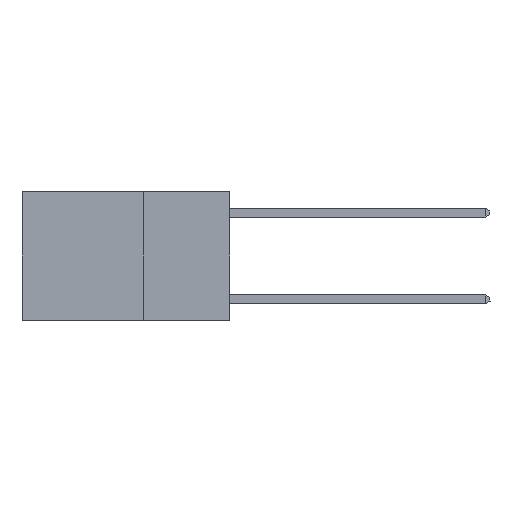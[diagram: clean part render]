
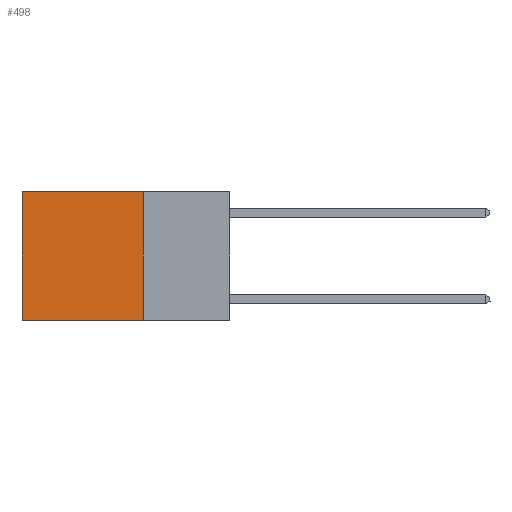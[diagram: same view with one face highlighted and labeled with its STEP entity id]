
A CAD part, left-side view. The second image highlights one B-rep face of the part: STEP entity #498.
In plain terms, the highlighted planar face has unit normal (-1, 0, 0).
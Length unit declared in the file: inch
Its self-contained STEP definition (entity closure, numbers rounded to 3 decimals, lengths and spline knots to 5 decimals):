
#197 = DIRECTION ( 'NONE',  ( 0., 1., 0. ) ) ;
#498 = ADVANCED_FACE ( 'NONE', ( #17595 ), #15581, .F. ) ;
#2174 = EDGE_CURVE ( 'NONE', #12027, #7402, #4754, .T. ) ;
#3318 = LINE ( 'NONE', #11327, #19541 ) ;
#3967 = ORIENTED_EDGE ( 'NONE', *, *, #12951, .T. ) ;
#4261 = VECTOR ( 'NONE', #20274, 39.37008 ) ;
#4628 = VERTEX_POINT ( 'NONE', #7171 ) ;
#4754 = LINE ( 'NONE', #18707, #4261 ) ;
#5888 = AXIS2_PLACEMENT_3D ( 'NONE', #7722, #9284, #20258 ) ;
#7171 = CARTESIAN_POINT ( 'NONE',  ( 0.2625, 0.6, -0.37 ) ) ;
#7172 = VERTEX_POINT ( 'NONE', #12004 ) ;
#7402 = VERTEX_POINT ( 'NONE', #12415 ) ;
#7722 = CARTESIAN_POINT ( 'NONE',  ( 0.2625, 0.25, 0. ) ) ;
#7856 = LINE ( 'NONE', #9628, #12034 ) ;
#8033 = EDGE_CURVE ( 'NONE', #7402, #4628, #13381, .T. ) ;
#9284 = DIRECTION ( 'NONE',  ( 1., 0., 0. ) ) ;
#9628 = CARTESIAN_POINT ( 'NONE',  ( 0.2625, 0.25, 0. ) ) ;
#10225 = CARTESIAN_POINT ( 'NONE',  ( 0.2625, 0.25, 0. ) ) ;
#11327 = CARTESIAN_POINT ( 'NONE',  ( 0.2625, 0.6, 0. ) ) ;
#12004 = CARTESIAN_POINT ( 'NONE',  ( 0.2625, 0.6, 0. ) ) ;
#12027 = VERTEX_POINT ( 'NONE', #10225 ) ;
#12034 = VECTOR ( 'NONE', #197, 39.37008 ) ;
#12415 = CARTESIAN_POINT ( 'NONE',  ( 0.2625, 0.25, -0.37 ) ) ;
#12887 = VECTOR ( 'NONE', #18996, 39.37008 ) ;
#12918 = DIRECTION ( 'NONE',  ( 0., 0., -1. ) ) ;
#12951 = EDGE_CURVE ( 'NONE', #12027, #7172, #7856, .T. ) ;
#13264 = EDGE_LOOP ( 'NONE', ( #16464, #17131, #16412, #3967 ) ) ;
#13381 = LINE ( 'NONE', #14298, #12887 ) ;
#14298 = CARTESIAN_POINT ( 'NONE',  ( 0.2625, 0.25, -0.37 ) ) ;
#15167 = EDGE_CURVE ( 'NONE', #7172, #4628, #3318, .T. ) ;
#15581 = PLANE ( 'NONE',  #5888 ) ;
#16412 = ORIENTED_EDGE ( 'NONE', *, *, #2174, .F. ) ;
#16464 = ORIENTED_EDGE ( 'NONE', *, *, #15167, .T. ) ;
#17131 = ORIENTED_EDGE ( 'NONE', *, *, #8033, .F. ) ;
#17595 = FACE_OUTER_BOUND ( 'NONE', #13264, .T. ) ;
#18707 = CARTESIAN_POINT ( 'NONE',  ( 0.2625, 0.25, 0. ) ) ;
#18996 = DIRECTION ( 'NONE',  ( 0., 1., 0. ) ) ;
#19541 = VECTOR ( 'NONE', #12918, 39.37008 ) ;
#20258 = DIRECTION ( 'NONE',  ( 0., 0., -1. ) ) ;
#20274 = DIRECTION ( 'NONE',  ( 0., 0., -1. ) ) ;
